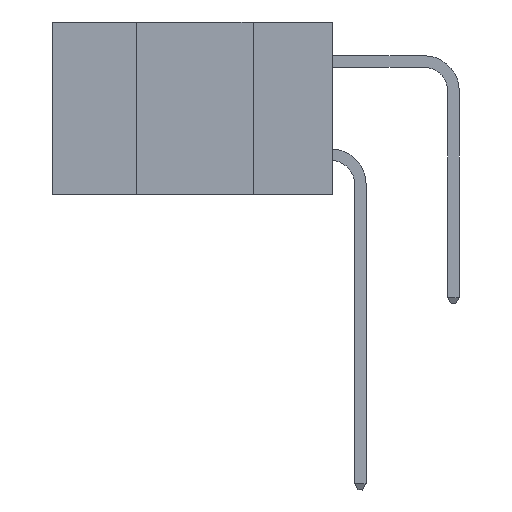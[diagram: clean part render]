
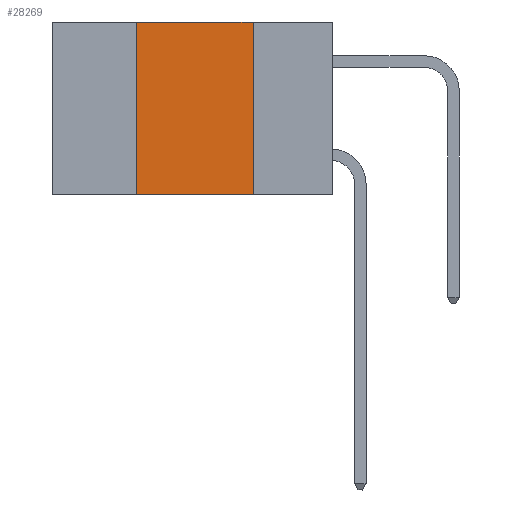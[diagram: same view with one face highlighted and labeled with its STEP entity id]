
A CAD part, left-side view. The second image highlights one B-rep face of the part: STEP entity #28269.
In plain terms, the highlighted planar face has unit normal (-1, 0, 0).
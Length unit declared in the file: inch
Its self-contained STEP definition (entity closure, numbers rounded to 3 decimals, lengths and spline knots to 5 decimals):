
#90 = AXIS2_PLACEMENT_3D ( 'NONE', #1389, #25554, #2973 ) ;
#573 = ORIENTED_EDGE ( 'NONE', *, *, #3531, .F. ) ;
#1246 = CARTESIAN_POINT ( 'NONE',  ( 0., 0.42, -0.37 ) ) ;
#1389 = CARTESIAN_POINT ( 'NONE',  ( 0., 0.6, 0. ) ) ;
#1404 = CARTESIAN_POINT ( 'NONE',  ( 0., 0.6, 0. ) ) ;
#2973 = DIRECTION ( 'NONE',  ( 0., 0., -1. ) ) ;
#3187 = ORIENTED_EDGE ( 'NONE', *, *, #6705, .T. ) ;
#3531 = EDGE_CURVE ( 'NONE', #12616, #17250, #21361, .T. ) ;
#3618 = ORIENTED_EDGE ( 'NONE', *, *, #27246, .F. ) ;
#6379 = CARTESIAN_POINT ( 'NONE',  ( 0., 0.6, -0.37 ) ) ;
#6460 = EDGE_CURVE ( 'NONE', #16399, #12616, #7447, .T. ) ;
#6705 = EDGE_CURVE ( 'NONE', #16399, #16405, #19538, .T. ) ;
#7447 = LINE ( 'NONE', #14390, #9938 ) ;
#8399 = DIRECTION ( 'NONE',  ( 0., -1., 0. ) ) ;
#9692 = LINE ( 'NONE', #13477, #23625 ) ;
#9917 = PLANE ( 'NONE',  #90 ) ;
#9938 = VECTOR ( 'NONE', #27732, 39.37008 ) ;
#10070 = CARTESIAN_POINT ( 'NONE',  ( 0., 0.17, -0.37 ) ) ;
#12616 = VERTEX_POINT ( 'NONE', #16956 ) ;
#13477 = CARTESIAN_POINT ( 'NONE',  ( 0., 0.17, -0.37 ) ) ;
#14390 = CARTESIAN_POINT ( 'NONE',  ( 0., 0.42, -0.37 ) ) ;
#16341 = DIRECTION ( 'NONE',  ( 0., 0., -1. ) ) ;
#16399 = VERTEX_POINT ( 'NONE', #1246 ) ;
#16405 = VERTEX_POINT ( 'NONE', #10070 ) ;
#16956 = CARTESIAN_POINT ( 'NONE',  ( 0., 0.42, 0. ) ) ;
#17250 = VERTEX_POINT ( 'NONE', #27410 ) ;
#18703 = VECTOR ( 'NONE', #27764, 39.37008 ) ;
#19538 = LINE ( 'NONE', #6379, #28014 ) ;
#20060 = EDGE_LOOP ( 'NONE', ( #3618, #573, #25418, #3187 ) ) ;
#21361 = LINE ( 'NONE', #1404, #18703 ) ;
#23625 = VECTOR ( 'NONE', #16341, 39.37008 ) ;
#25117 = FACE_OUTER_BOUND ( 'NONE', #20060, .T. ) ;
#25418 = ORIENTED_EDGE ( 'NONE', *, *, #6460, .F. ) ;
#25554 = DIRECTION ( 'NONE',  ( 1., 0., 0. ) ) ;
#27246 = EDGE_CURVE ( 'NONE', #17250, #16405, #9692, .T. ) ;
#27410 = CARTESIAN_POINT ( 'NONE',  ( 0., 0.17, 0. ) ) ;
#27732 = DIRECTION ( 'NONE',  ( 0., 0., 1. ) ) ;
#27764 = DIRECTION ( 'NONE',  ( 0., -1., 0. ) ) ;
#28014 = VECTOR ( 'NONE', #8399, 39.37008 ) ;
#28269 = ADVANCED_FACE ( 'NONE', ( #25117 ), #9917, .F. ) ;
